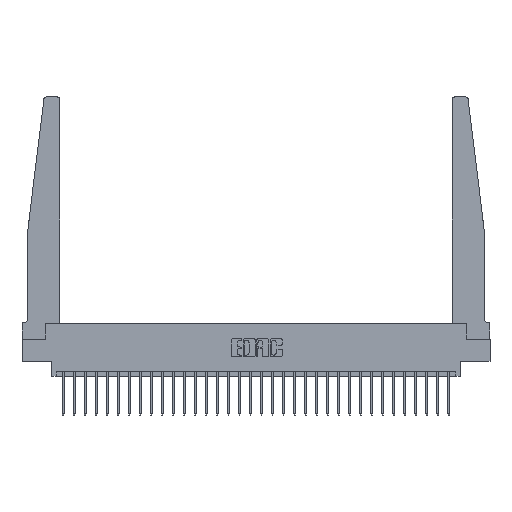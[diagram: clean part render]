
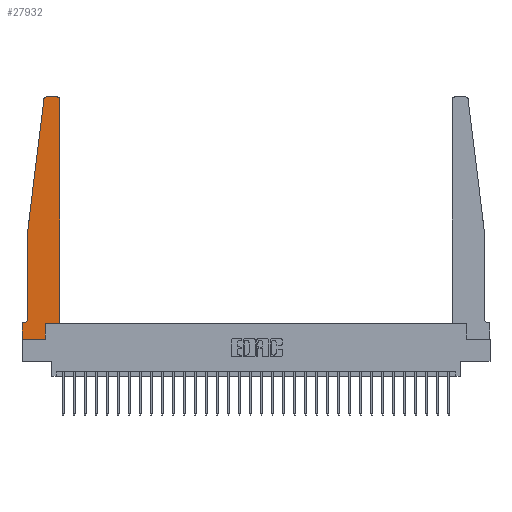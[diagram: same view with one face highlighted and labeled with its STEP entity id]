
A CAD part, top view. The second image highlights one B-rep face of the part: STEP entity #27932.
In plain terms, the highlighted planar face has unit normal (0, 0, 1).
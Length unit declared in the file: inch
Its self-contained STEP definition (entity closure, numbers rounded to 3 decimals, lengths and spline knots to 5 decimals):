
#4 = EDGE_CURVE ( 'NONE', #23674, #20522, #19946, .T. ) ;
#418 = EDGE_CURVE ( 'NONE', #15792, #11215, #2700, .T. ) ;
#754 = AXIS2_PLACEMENT_3D ( 'NONE', #5587, #24004, #21469 ) ;
#1334 = DIRECTION ( 'NONE',  ( 0., 0., 1. ) ) ;
#1542 = EDGE_CURVE ( 'NONE', #20932, #28011, #15232, .T. ) ;
#1795 = DIRECTION ( 'NONE',  ( -1., 0., 0. ) ) ;
#1796 = VECTOR ( 'NONE', #8498, 39.37008 ) ;
#2176 = ORIENTED_EDGE ( 'NONE', *, *, #11193, .T. ) ;
#2188 = DIRECTION ( 'NONE',  ( 1., 0., 0. ) ) ;
#2371 = DIRECTION ( 'NONE',  ( -1., 0., 0. ) ) ;
#2700 = CIRCLE ( 'NONE', #754, 0.03 ) ;
#2980 = CARTESIAN_POINT ( 'NONE',  ( 0.395, 2.75, 0.37 ) ) ;
#3104 = CARTESIAN_POINT ( 'NONE',  ( 0.425, 0.18, 0.37 ) ) ;
#3163 = LINE ( 'NONE', #9483, #8440 ) ;
#3693 = CARTESIAN_POINT ( 'NONE',  ( 0.065, 1.25, 0.37 ) ) ;
#4179 = CARTESIAN_POINT ( 'NONE',  ( 0.065, 1.25, 0.37 ) ) ;
#5587 = CARTESIAN_POINT ( 'NONE',  ( 0.395, 2.72, 0.37 ) ) ;
#5757 = LINE ( 'NONE', #12625, #25603 ) ;
#7948 = FACE_OUTER_BOUND ( 'NONE', #26535, .T. ) ;
#8263 = CARTESIAN_POINT ( 'NONE',  ( 0.2605, 0.18, 0.37 ) ) ;
#8440 = VECTOR ( 'NONE', #16354, 39.37008 ) ;
#8455 = DIRECTION ( 'NONE',  ( 0., 1., 0. ) ) ;
#8498 = DIRECTION ( 'NONE',  ( 0., -1., 0. ) ) ;
#8540 = DIRECTION ( 'NONE',  ( -0.122, -0.992, 0. ) ) ;
#8715 = CARTESIAN_POINT ( 'NONE',  ( 0.2605, 0.18, 0.37 ) ) ;
#8852 = CARTESIAN_POINT ( 'NONE',  ( 0.425, 0.18, 0.37 ) ) ;
#8985 = CARTESIAN_POINT ( 'NONE',  ( 0.065, 1.25, 0.37 ) ) ;
#9372 = CARTESIAN_POINT ( 'NONE',  ( 0.065, 0.2375, 0.37 ) ) ;
#9483 = CARTESIAN_POINT ( 'NONE',  ( 0., 0., 0.37 ) ) ;
#9976 = EDGE_CURVE ( 'NONE', #28011, #23590, #24720, .T. ) ;
#10084 = CARTESIAN_POINT ( 'NONE',  ( 0., 0., 0.37 ) ) ;
#10443 = VERTEX_POINT ( 'NONE', #19719 ) ;
#10490 = ORIENTED_EDGE ( 'NONE', *, *, #22246, .T. ) ;
#10524 = ORIENTED_EDGE ( 'NONE', *, *, #17800, .T. ) ;
#10608 = VECTOR ( 'NONE', #2371, 39.37008 ) ;
#10652 = DIRECTION ( 'NONE',  ( 0., 0., -1. ) ) ;
#11193 = EDGE_CURVE ( 'NONE', #11215, #20932, #29579, .T. ) ;
#11215 = VERTEX_POINT ( 'NONE', #2980 ) ;
#12075 = ORIENTED_EDGE ( 'NONE', *, *, #9976, .T. ) ;
#12516 = ORIENTED_EDGE ( 'NONE', *, *, #21423, .T. ) ;
#12625 = CARTESIAN_POINT ( 'NONE',  ( 0.425, 0.18, 0.37 ) ) ;
#12819 = VERTEX_POINT ( 'NONE', #15984 ) ;
#13119 = LINE ( 'NONE', #3693, #1796 ) ;
#13484 = DIRECTION ( 'NONE',  ( 1., 0., 0. ) ) ;
#13916 = VECTOR ( 'NONE', #26394, 39.37008 ) ;
#14007 = ORIENTED_EDGE ( 'NONE', *, *, #4, .T. ) ;
#14576 = CARTESIAN_POINT ( 'NONE',  ( 0.425, 2.72, 0.37 ) ) ;
#14627 = ORIENTED_EDGE ( 'NONE', *, *, #25050, .T. ) ;
#14730 = VECTOR ( 'NONE', #21465, 39.37008 ) ;
#15232 = CIRCLE ( 'NONE', #29146, 0.03 ) ;
#15331 = EDGE_CURVE ( 'NONE', #20522, #25217, #29409, .T. ) ;
#15484 = VECTOR ( 'NONE', #28968, 39.37008 ) ;
#15792 = VERTEX_POINT ( 'NONE', #14576 ) ;
#15984 = CARTESIAN_POINT ( 'NONE',  ( 0., 0.1875, 0.37 ) ) ;
#16354 = DIRECTION ( 'NONE',  ( 1., 0., 0. ) ) ;
#16470 = VECTOR ( 'NONE', #13484, 39.37008 ) ;
#17076 = CARTESIAN_POINT ( 'NONE',  ( 0., 0.1875, 0.37 ) ) ;
#17800 = EDGE_CURVE ( 'NONE', #22335, #10443, #25663, .T. ) ;
#18144 = CARTESIAN_POINT ( 'NONE',  ( 0.25, 2.75, 0.37 ) ) ;
#18251 = CARTESIAN_POINT ( 'NONE',  ( 0.065, 0.1875, 0.37 ) ) ;
#18845 = ORIENTED_EDGE ( 'NONE', *, *, #418, .T. ) ;
#19016 = CARTESIAN_POINT ( 'NONE',  ( 0.24675, 2.72367, 0.37 ) ) ;
#19226 = AXIS2_PLACEMENT_3D ( 'NONE', #17076, #1334, #26258 ) ;
#19719 = CARTESIAN_POINT ( 'NONE',  ( 0.015, 0.1875, 0.37 ) ) ;
#19946 = LINE ( 'NONE', #8715, #15484 ) ;
#20323 = DIRECTION ( 'NONE',  ( 0., 0., 1. ) ) ;
#20522 = VERTEX_POINT ( 'NONE', #8263 ) ;
#20753 = CARTESIAN_POINT ( 'NONE',  ( 0., 0., 0.37 ) ) ;
#20932 = VERTEX_POINT ( 'NONE', #22259 ) ;
#21083 = VERTEX_POINT ( 'NONE', #20753 ) ;
#21423 = EDGE_CURVE ( 'NONE', #25217, #15792, #5757, .T. ) ;
#21465 = DIRECTION ( 'NONE',  ( 0., -1., 0. ) ) ;
#21469 = DIRECTION ( 'NONE',  ( 1., 0., 0. ) ) ;
#21672 = EDGE_CURVE ( 'NONE', #21083, #23674, #3163, .T. ) ;
#22246 = EDGE_CURVE ( 'NONE', #23590, #22335, #13119, .T. ) ;
#22259 = CARTESIAN_POINT ( 'NONE',  ( 0.27653, 2.75, 0.37 ) ) ;
#22285 = AXIS2_PLACEMENT_3D ( 'NONE', #26858, #10652, #1795 ) ;
#22335 = VERTEX_POINT ( 'NONE', #9372 ) ;
#22942 = EDGE_CURVE ( 'NONE', #12819, #21083, #23251, .T. ) ;
#23157 = CARTESIAN_POINT ( 'NONE',  ( 0.27653, 2.72, 0.37 ) ) ;
#23181 = CARTESIAN_POINT ( 'NONE',  ( 0.2605, 0., 0.37 ) ) ;
#23251 = LINE ( 'NONE', #10084, #14730 ) ;
#23590 = VERTEX_POINT ( 'NONE', #8985 ) ;
#23614 = ORIENTED_EDGE ( 'NONE', *, *, #15331, .T. ) ;
#23674 = VERTEX_POINT ( 'NONE', #23181 ) ;
#24004 = DIRECTION ( 'NONE',  ( 0., 0., 1. ) ) ;
#24286 = PLANE ( 'NONE',  #19226 ) ;
#24720 = LINE ( 'NONE', #4179, #29001 ) ;
#25050 = EDGE_CURVE ( 'NONE', #10443, #12819, #27440, .T. ) ;
#25175 = ORIENTED_EDGE ( 'NONE', *, *, #21672, .T. ) ;
#25217 = VERTEX_POINT ( 'NONE', #3104 ) ;
#25603 = VECTOR ( 'NONE', #8455, 39.37008 ) ;
#25663 = CIRCLE ( 'NONE', #22285, 0.05 ) ;
#26258 = DIRECTION ( 'NONE',  ( 1., 0., 0. ) ) ;
#26394 = DIRECTION ( 'NONE',  ( -1., 0., 0. ) ) ;
#26535 = EDGE_LOOP ( 'NONE', ( #2176, #29335, #12075, #10490, #10524, #14627, #28981, #25175, #14007, #23614, #12516, #18845 ) ) ;
#26858 = CARTESIAN_POINT ( 'NONE',  ( 0.015, 0.2375, 0.37 ) ) ;
#27440 = LINE ( 'NONE', #18251, #10608 ) ;
#27932 = ADVANCED_FACE ( 'NONE', ( #7948 ), #24286, .T. ) ;
#28011 = VERTEX_POINT ( 'NONE', #19016 ) ;
#28968 = DIRECTION ( 'NONE',  ( 0., 1., 0. ) ) ;
#28981 = ORIENTED_EDGE ( 'NONE', *, *, #22942, .T. ) ;
#29001 = VECTOR ( 'NONE', #8540, 39.37008 ) ;
#29146 = AXIS2_PLACEMENT_3D ( 'NONE', #23157, #20323, #2188 ) ;
#29335 = ORIENTED_EDGE ( 'NONE', *, *, #1542, .T. ) ;
#29409 = LINE ( 'NONE', #8852, #16470 ) ;
#29579 = LINE ( 'NONE', #18144, #13916 ) ;
